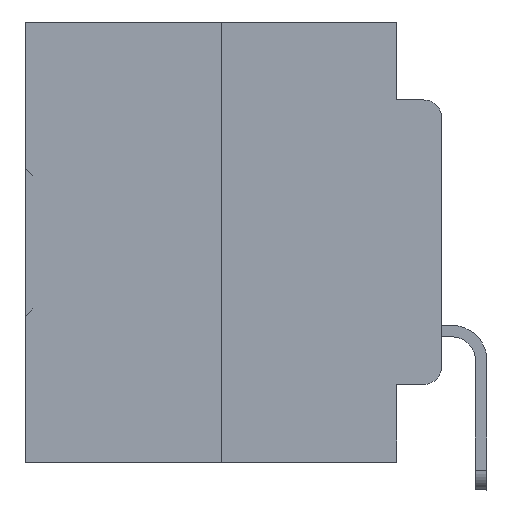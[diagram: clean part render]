
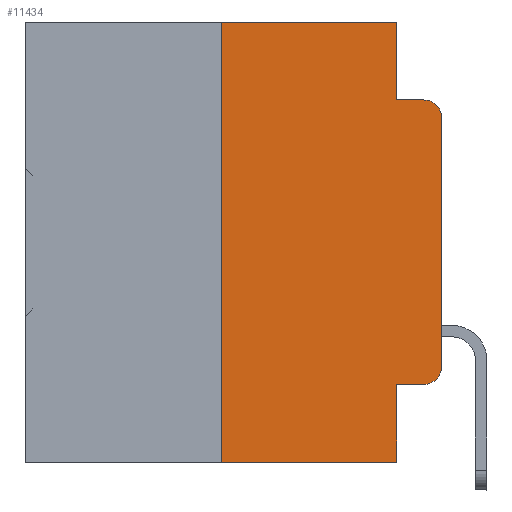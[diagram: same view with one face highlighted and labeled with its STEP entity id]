
A CAD part, left-side view. The second image highlights one B-rep face of the part: STEP entity #11434.
In plain terms, the highlighted planar face has unit normal (-1, 0, 0).
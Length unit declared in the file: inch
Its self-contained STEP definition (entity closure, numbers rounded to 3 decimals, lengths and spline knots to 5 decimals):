
#1221 = CARTESIAN_POINT ( 'NONE',  ( 0., 0.02, -0.1085 ) ) ;
#1603 = VERTEX_POINT ( 'NONE', #33157 ) ;
#2088 = DIRECTION ( 'NONE',  ( 0., 0., -1. ) ) ;
#2257 = FACE_OUTER_BOUND ( 'NONE', #29814, .T. ) ;
#3581 = CARTESIAN_POINT ( 'NONE',  ( 0., 0.02, -0.0885 ) ) ;
#3630 = LINE ( 'NONE', #30205, #35053 ) ;
#4109 = VECTOR ( 'NONE', #17199, 39.37008 ) ;
#4906 = ORIENTED_EDGE ( 'NONE', *, *, #14470, .T. ) ;
#4954 = EDGE_CURVE ( 'NONE', #25457, #15058, #18519, .T. ) ;
#5168 = ORIENTED_EDGE ( 'NONE', *, *, #5534, .F. ) ;
#5352 = VECTOR ( 'NONE', #13633, 39.37008 ) ;
#5404 = LINE ( 'NONE', #16953, #4109 ) ;
#5518 = ORIENTED_EDGE ( 'NONE', *, *, #29485, .T. ) ;
#5534 = EDGE_CURVE ( 'NONE', #5669, #17542, #26751, .T. ) ;
#5669 = VERTEX_POINT ( 'NONE', #8996 ) ;
#5797 = ORIENTED_EDGE ( 'NONE', *, *, #10863, .F. ) ;
#5859 = CARTESIAN_POINT ( 'NONE',  ( 0., 0.473, 0. ) ) ;
#6277 = EDGE_CURVE ( 'NONE', #15058, #17542, #12223, .T. ) ;
#6758 = DIRECTION ( 'NONE',  ( 0., 0., 1. ) ) ;
#6954 = EDGE_CURVE ( 'NONE', #1603, #10669, #31920, .T. ) ;
#7416 = DIRECTION ( 'NONE',  ( 0., 0., -1. ) ) ;
#7772 = DIRECTION ( 'NONE',  ( -1., 0., 0. ) ) ;
#7836 = DIRECTION ( 'NONE',  ( 0., -1., 0. ) ) ;
#8276 = CARTESIAN_POINT ( 'NONE',  ( 0., 0.02, -0.4115 ) ) ;
#8414 = CARTESIAN_POINT ( 'NONE',  ( 0., 0.051, -0.0885 ) ) ;
#8996 = CARTESIAN_POINT ( 'NONE',  ( 0., 0.051, -0.0885 ) ) ;
#10448 = DIRECTION ( 'NONE',  ( 0., -1., 0. ) ) ;
#10669 = VERTEX_POINT ( 'NONE', #27889 ) ;
#10680 = CARTESIAN_POINT ( 'NONE',  ( 0., 0.473, -0.5 ) ) ;
#10863 = EDGE_CURVE ( 'NONE', #29146, #35830, #3630, .T. ) ;
#11434 = ADVANCED_FACE ( 'NONE', ( #2257 ), #36129, .F. ) ;
#11461 = CARTESIAN_POINT ( 'NONE',  ( 0., 0., -0.3915 ) ) ;
#12045 = LINE ( 'NONE', #32492, #14224 ) ;
#12197 = ORIENTED_EDGE ( 'NONE', *, *, #4954, .T. ) ;
#12223 = CIRCLE ( 'NONE', #15577, 0.02 ) ;
#13633 = DIRECTION ( 'NONE',  ( 0., -1., 0. ) ) ;
#14224 = VECTOR ( 'NONE', #7416, 39.37008 ) ;
#14273 = CARTESIAN_POINT ( 'NONE',  ( 0., 0.051, 0. ) ) ;
#14470 = EDGE_CURVE ( 'NONE', #29146, #18571, #26926, .T. ) ;
#14575 = CIRCLE ( 'NONE', #24252, 0.02 ) ;
#14772 = VERTEX_POINT ( 'NONE', #14273 ) ;
#14833 = ORIENTED_EDGE ( 'NONE', *, *, #6277, .T. ) ;
#15058 = VERTEX_POINT ( 'NONE', #21478 ) ;
#15577 = AXIS2_PLACEMENT_3D ( 'NONE', #1221, #34731, #18043 ) ;
#16021 = EDGE_CURVE ( 'NONE', #10669, #14772, #5404, .T. ) ;
#16256 = DIRECTION ( 'NONE',  ( 0., 0., -1. ) ) ;
#16620 = ORIENTED_EDGE ( 'NONE', *, *, #16021, .F. ) ;
#16733 = DIRECTION ( 'NONE',  ( 1., 0., 0. ) ) ;
#16953 = CARTESIAN_POINT ( 'NONE',  ( 0., 0.473, 0. ) ) ;
#17199 = DIRECTION ( 'NONE',  ( 0., -1., 0. ) ) ;
#17542 = VERTEX_POINT ( 'NONE', #3581 ) ;
#18043 = DIRECTION ( 'NONE',  ( 0., 0., -1. ) ) ;
#18519 = LINE ( 'NONE', #27888, #23314 ) ;
#18571 = VERTEX_POINT ( 'NONE', #8276 ) ;
#20122 = VECTOR ( 'NONE', #6758, 39.37008 ) ;
#20328 = CARTESIAN_POINT ( 'NONE',  ( 0., 0.25, 0. ) ) ;
#21121 = ORIENTED_EDGE ( 'NONE', *, *, #6954, .F. ) ;
#21478 = CARTESIAN_POINT ( 'NONE',  ( 0., 0., -0.1085 ) ) ;
#22462 = ORIENTED_EDGE ( 'NONE', *, *, #26284, .F. ) ;
#23314 = VECTOR ( 'NONE', #30346, 39.37008 ) ;
#23456 = CARTESIAN_POINT ( 'NONE',  ( 0., 0.051, -0.4115 ) ) ;
#24252 = AXIS2_PLACEMENT_3D ( 'NONE', #24542, #7772, #2088 ) ;
#24542 = CARTESIAN_POINT ( 'NONE',  ( 0., 0.02, -0.3915 ) ) ;
#25206 = VECTOR ( 'NONE', #7836, 39.37008 ) ;
#25457 = VERTEX_POINT ( 'NONE', #11461 ) ;
#26284 = EDGE_CURVE ( 'NONE', #14772, #5669, #12045, .T. ) ;
#26649 = VECTOR ( 'NONE', #10448, 39.37008 ) ;
#26751 = LINE ( 'NONE', #8414, #5352 ) ;
#26926 = LINE ( 'NONE', #29844, #25206 ) ;
#26950 = ORIENTED_EDGE ( 'NONE', *, *, #35794, .T. ) ;
#27888 = CARTESIAN_POINT ( 'NONE',  ( 0., 0., 0. ) ) ;
#27889 = CARTESIAN_POINT ( 'NONE',  ( 0., 0.25, 0. ) ) ;
#29146 = VERTEX_POINT ( 'NONE', #23456 ) ;
#29345 = AXIS2_PLACEMENT_3D ( 'NONE', #5859, #16733, #33797 ) ;
#29485 = EDGE_CURVE ( 'NONE', #1603, #35830, #31470, .T. ) ;
#29814 = EDGE_LOOP ( 'NONE', ( #12197, #14833, #5168, #22462, #16620, #21121, #5518, #5797, #4906, #26950 ) ) ;
#29844 = CARTESIAN_POINT ( 'NONE',  ( 0., 0.051, -0.4115 ) ) ;
#30205 = CARTESIAN_POINT ( 'NONE',  ( 0., 0.051, 0. ) ) ;
#30346 = DIRECTION ( 'NONE',  ( 0., 0., 1. ) ) ;
#31470 = LINE ( 'NONE', #10680, #26649 ) ;
#31920 = LINE ( 'NONE', #20328, #20122 ) ;
#32492 = CARTESIAN_POINT ( 'NONE',  ( 0., 0.051, 0. ) ) ;
#33157 = CARTESIAN_POINT ( 'NONE',  ( 0., 0.25, -0.5 ) ) ;
#33797 = DIRECTION ( 'NONE',  ( 0., 0., -1. ) ) ;
#34731 = DIRECTION ( 'NONE',  ( -1., 0., 0. ) ) ;
#35053 = VECTOR ( 'NONE', #16256, 39.37008 ) ;
#35512 = CARTESIAN_POINT ( 'NONE',  ( 0., 0.051, -0.5 ) ) ;
#35794 = EDGE_CURVE ( 'NONE', #18571, #25457, #14575, .T. ) ;
#35830 = VERTEX_POINT ( 'NONE', #35512 ) ;
#36129 = PLANE ( 'NONE',  #29345 ) ;
